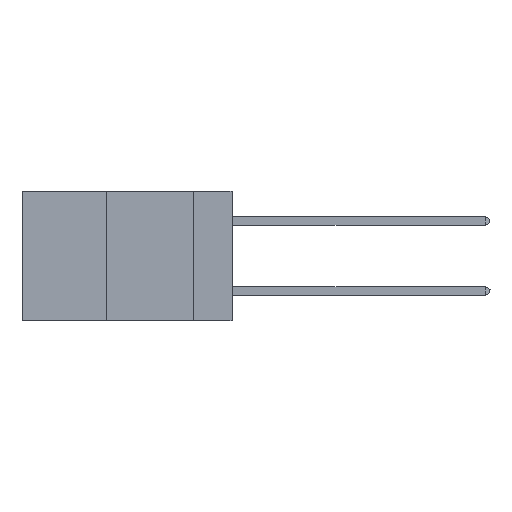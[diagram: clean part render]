
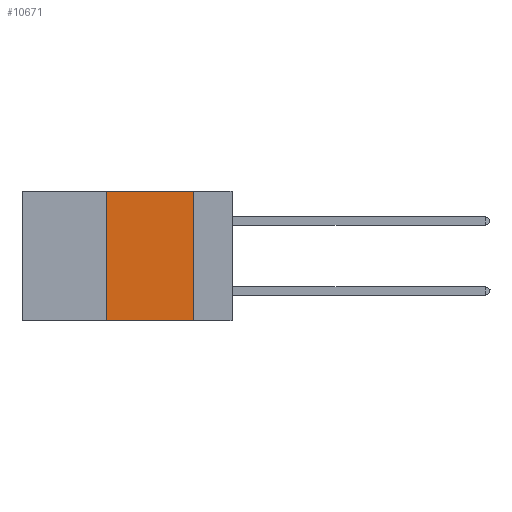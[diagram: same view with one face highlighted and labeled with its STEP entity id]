
A CAD part, left-side view. The second image highlights one B-rep face of the part: STEP entity #10671.
In plain terms, the highlighted planar face has unit normal (-1, 0, 0).
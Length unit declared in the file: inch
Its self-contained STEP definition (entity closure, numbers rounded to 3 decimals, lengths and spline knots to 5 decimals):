
#258 = VERTEX_POINT ( 'NONE', #20793 ) ;
#481 = CARTESIAN_POINT ( 'NONE',  ( 0., 0.6, 0. ) ) ;
#2249 = EDGE_CURVE ( 'NONE', #258, #3993, #2764, .T. ) ;
#2446 = EDGE_CURVE ( 'NONE', #3993, #18742, #11672, .T. ) ;
#2764 = LINE ( 'NONE', #481, #12547 ) ;
#3560 = FACE_OUTER_BOUND ( 'NONE', #20073, .T. ) ;
#3993 = VERTEX_POINT ( 'NONE', #17184 ) ;
#3995 = CARTESIAN_POINT ( 'NONE',  ( 0., 0.6, 0. ) ) ;
#5125 = DIRECTION ( 'NONE',  ( 0., 0., -1. ) ) ;
#5197 = DIRECTION ( 'NONE',  ( 0., -1., 0. ) ) ;
#7881 = ORIENTED_EDGE ( 'NONE', *, *, #2249, .F. ) ;
#10671 = ADVANCED_FACE ( 'NONE', ( #3560 ), #10868, .F. ) ;
#10868 = PLANE ( 'NONE',  #24997 ) ;
#11672 = LINE ( 'NONE', #21423, #22287 ) ;
#11905 = DIRECTION ( 'NONE',  ( 0., -1., 0. ) ) ;
#12547 = VECTOR ( 'NONE', #5197, 39.37008 ) ;
#12684 = DIRECTION ( 'NONE',  ( 1., 0., 0. ) ) ;
#14177 = LINE ( 'NONE', #23482, #19468 ) ;
#16020 = ORIENTED_EDGE ( 'NONE', *, *, #23205, .T. ) ;
#16122 = ORIENTED_EDGE ( 'NONE', *, *, #19509, .F. ) ;
#17184 = CARTESIAN_POINT ( 'NONE',  ( 0., 0.11, 0. ) ) ;
#18033 = CARTESIAN_POINT ( 'NONE',  ( 0., 0.36, -0.37 ) ) ;
#18742 = VERTEX_POINT ( 'NONE', #29533 ) ;
#19468 = VECTOR ( 'NONE', #11905, 39.37008 ) ;
#19509 = EDGE_CURVE ( 'NONE', #28319, #258, #27007, .T. ) ;
#20020 = ORIENTED_EDGE ( 'NONE', *, *, #2446, .F. ) ;
#20073 = EDGE_LOOP ( 'NONE', ( #20020, #7881, #16122, #16020 ) ) ;
#20137 = DIRECTION ( 'NONE',  ( 0., 0., 1. ) ) ;
#20793 = CARTESIAN_POINT ( 'NONE',  ( 0., 0.36, 0. ) ) ;
#21423 = CARTESIAN_POINT ( 'NONE',  ( 0., 0.11, 0. ) ) ;
#21566 = VECTOR ( 'NONE', #20137, 39.37008 ) ;
#22156 = DIRECTION ( 'NONE',  ( 0., 0., -1. ) ) ;
#22287 = VECTOR ( 'NONE', #5125, 39.37008 ) ;
#23205 = EDGE_CURVE ( 'NONE', #28319, #18742, #14177, .T. ) ;
#23482 = CARTESIAN_POINT ( 'NONE',  ( 0., 0.6, -0.37 ) ) ;
#24997 = AXIS2_PLACEMENT_3D ( 'NONE', #3995, #12684, #22156 ) ;
#27007 = LINE ( 'NONE', #27148, #21566 ) ;
#27148 = CARTESIAN_POINT ( 'NONE',  ( 0., 0.36, 0. ) ) ;
#28319 = VERTEX_POINT ( 'NONE', #18033 ) ;
#29533 = CARTESIAN_POINT ( 'NONE',  ( 0., 0.11, -0.37 ) ) ;
